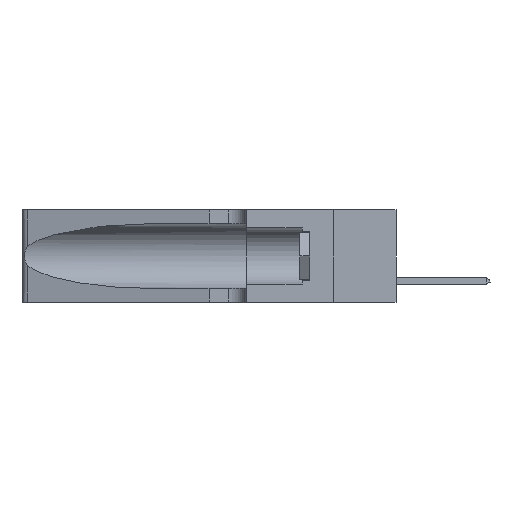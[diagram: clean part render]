
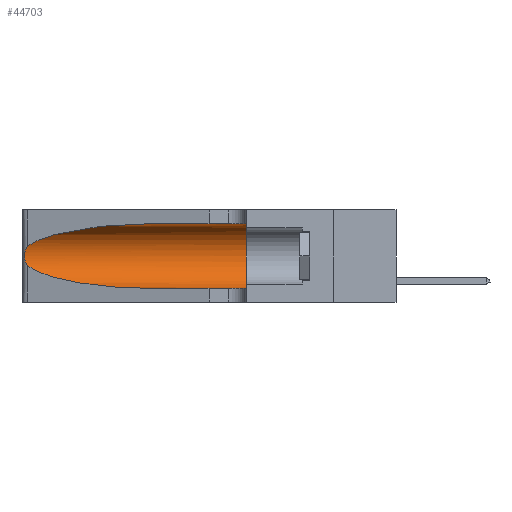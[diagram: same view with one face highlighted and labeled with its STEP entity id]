
A CAD part, left-side view. The second image highlights one B-rep face of the part: STEP entity #44703.
In plain terms, the highlighted cylindrical face has radius 3.308 mm (diameter 6.617 mm), a partial arc.
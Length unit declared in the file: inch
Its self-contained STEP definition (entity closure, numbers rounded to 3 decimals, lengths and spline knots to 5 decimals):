
#1345 = CARTESIAN_POINT ( 'NONE',  ( 0.1305, 1.61858, 0.31525 ) ) ;
#1456 = VECTOR ( 'NONE', #12982, 39.37008 ) ;
#1526 = LINE ( 'NONE', #47453, #8166 ) ;
#2474 = CARTESIAN_POINT ( 'NONE',  ( 0.18966, 0.96281, 0.05475 ) ) ;
#3058 = EDGE_CURVE ( 'NONE', #39833, #16531, #39866, .T. ) ;
#3424 = CARTESIAN_POINT ( 'NONE',  ( 0.26075, 1.23896, 0.19203 ) ) ;
#3947 = CARTESIAN_POINT ( 'NONE',  ( 0.1305, 0.35, 0.31525 ) ) ;
#3964 =( BOUNDED_CURVE ( )  B_SPLINE_CURVE ( 3, ( #33875, #34039, #11631, #26114 ),
 .UNSPECIFIED., .F., .F. ) 
 B_SPLINE_CURVE_WITH_KNOTS ( ( 4, 4 ),
 ( 1.5708, 2.84003 ),
 .UNSPECIFIED. ) 
 CURVE ( )  GEOMETRIC_REPRESENTATION_ITEM ( )  RATIONAL_B_SPLINE_CURVE ( ( 1., 0.87, 0.87, 1. ) ) 
 REPRESENTATION_ITEM ( '' )  );
#5679 = VERTEX_POINT ( 'NONE', #9797 ) ;
#6793 = FACE_OUTER_BOUND ( 'NONE', #22926, .T. ) ;
#7831 = CARTESIAN_POINT ( 'NONE',  ( 0.25787, 1.23484, 0.2124 ) ) ;
#8166 = VECTOR ( 'NONE', #40306, 39.37008 ) ;
#9797 = CARTESIAN_POINT ( 'NONE',  ( 0.1305, 0.72297, 0.31525 ) ) ;
#9865 = VERTEX_POINT ( 'NONE', #22354 ) ;
#11631 = CARTESIAN_POINT ( 'NONE',  ( 0.2373, 1.15595, 0.28018 ) ) ;
#11641 = CARTESIAN_POINT ( 'NONE',  ( 0.25854, 1.2359, 0.20912 ) ) ;
#11801 = CARTESIAN_POINT ( 'NONE',  ( 0.25555, 1.22993, 0.14849 ) ) ;
#12735 = CARTESIAN_POINT ( 'NONE',  ( 0.25487, 1.22718, 0.14631 ) ) ;
#12982 = DIRECTION ( 'NONE',  ( 0., -1., 0. ) ) ;
#15168 = DIRECTION ( 'NONE',  ( 0., 0., -1. ) ) ;
#15438 = CARTESIAN_POINT ( 'NONE',  ( 0.25789, 1.23486, 0.15765 ) ) ;
#15832 = VERTEX_POINT ( 'NONE', #45997 ) ;
#15910 = CARTESIAN_POINT ( 'NONE',  ( 0.26017, 1.23833, 0.17102 ) ) ;
#16397 = B_SPLINE_CURVE_WITH_KNOTS ( 'NONE', 3,
 ( #17649, #21635, #41900, #7831, #11641, #18788, #3424, #42201, #15910, #34995, #15438, #26889, #11801, #12735 ),
 .UNSPECIFIED., .F., .F.,
 ( 4, 2, 2, 2, 2, 2, 4 ),
 ( 0., 0.00027, 0.00053, 0.00107, 0.0016, 0.00187, 0.00214 ),
 .UNSPECIFIED. ) ;
#16531 = VERTEX_POINT ( 'NONE', #26432 ) ;
#16552 = CARTESIAN_POINT ( 'NONE',  ( 0.1305, 0.35, 0.185 ) ) ;
#16793 = CYLINDRICAL_SURFACE ( 'NONE', #22483, 0.13025 ) ;
#17649 = CARTESIAN_POINT ( 'NONE',  ( 0.25487, 1.22718, 0.22369 ) ) ;
#17921 =( BOUNDED_CURVE ( )  B_SPLINE_CURVE ( 3, ( #32791, #21204, #2474, #32284 ),
 .UNSPECIFIED., .F., .F. ) 
 B_SPLINE_CURVE_WITH_KNOTS ( ( 4, 4 ),
 ( 3.44316, 4.71239 ),
 .UNSPECIFIED. ) 
 CURVE ( )  GEOMETRIC_REPRESENTATION_ITEM ( )  RATIONAL_B_SPLINE_CURVE ( ( 1., 0.87, 0.87, 1. ) ) 
 REPRESENTATION_ITEM ( '' )  );
#18788 = CARTESIAN_POINT ( 'NONE',  ( 0.26018, 1.23835, 0.19895 ) ) ;
#19609 = EDGE_CURVE ( 'NONE', #5679, #15832, #3964, .T. ) ;
#20183 = VERTEX_POINT ( 'NONE', #21693 ) ;
#20194 = ORIENTED_EDGE ( 'NONE', *, *, #19609, .T. ) ;
#21204 = CARTESIAN_POINT ( 'NONE',  ( 0.2373, 1.15595, 0.08982 ) ) ;
#21635 = CARTESIAN_POINT ( 'NONE',  ( 0.25555, 1.22994, 0.2215 ) ) ;
#21693 = CARTESIAN_POINT ( 'NONE',  ( 0.1305, 0.72297, 0.05475 ) ) ;
#22354 = CARTESIAN_POINT ( 'NONE',  ( 0.25487, 1.22718, 0.14631 ) ) ;
#22483 = AXIS2_PLACEMENT_3D ( 'NONE', #34413, #46267, #15168 ) ;
#22926 = EDGE_LOOP ( 'NONE', ( #20194, #25824, #36470, #25529, #37662, #26844 ) ) ;
#25529 = ORIENTED_EDGE ( 'NONE', *, *, #39795, .T. ) ;
#25824 = ORIENTED_EDGE ( 'NONE', *, *, #34893, .T. ) ;
#26114 = CARTESIAN_POINT ( 'NONE',  ( 0.25487, 1.22718, 0.22369 ) ) ;
#26432 = CARTESIAN_POINT ( 'NONE',  ( 0.1305, 0.35, 0.05475 ) ) ;
#26844 = ORIENTED_EDGE ( 'NONE', *, *, #29515, .F. ) ;
#26889 = CARTESIAN_POINT ( 'NONE',  ( 0.25639, 1.23186, 0.15144 ) ) ;
#27024 = AXIS2_PLACEMENT_3D ( 'NONE', #16552, #31777, #46833 ) ;
#29515 = EDGE_CURVE ( 'NONE', #5679, #39833, #31720, .T. ) ;
#31720 = LINE ( 'NONE', #1345, #1456 ) ;
#31777 = DIRECTION ( 'NONE',  ( 0., 1., 0. ) ) ;
#32284 = CARTESIAN_POINT ( 'NONE',  ( 0.1305, 0.72297, 0.05475 ) ) ;
#32791 = CARTESIAN_POINT ( 'NONE',  ( 0.25487, 1.22718, 0.14631 ) ) ;
#33875 = CARTESIAN_POINT ( 'NONE',  ( 0.1305, 0.72297, 0.31525 ) ) ;
#34039 = CARTESIAN_POINT ( 'NONE',  ( 0.18966, 0.96281, 0.31525 ) ) ;
#34413 = CARTESIAN_POINT ( 'NONE',  ( 0.1305, 1.61858, 0.185 ) ) ;
#34893 = EDGE_CURVE ( 'NONE', #15832, #9865, #16397, .T. ) ;
#34995 = CARTESIAN_POINT ( 'NONE',  ( 0.25856, 1.23593, 0.16098 ) ) ;
#36470 = ORIENTED_EDGE ( 'NONE', *, *, #48882, .T. ) ;
#37662 = ORIENTED_EDGE ( 'NONE', *, *, #3058, .F. ) ;
#39795 = EDGE_CURVE ( 'NONE', #20183, #16531, #1526, .T. ) ;
#39833 = VERTEX_POINT ( 'NONE', #3947 ) ;
#39866 = CIRCLE ( 'NONE', #27024, 0.13025 ) ;
#40306 = DIRECTION ( 'NONE',  ( 0., -1., 0. ) ) ;
#41900 = CARTESIAN_POINT ( 'NONE',  ( 0.25639, 1.23184, 0.21858 ) ) ;
#42201 = CARTESIAN_POINT ( 'NONE',  ( 0.26075, 1.23896, 0.178 ) ) ;
#44703 = ADVANCED_FACE ( 'NONE', ( #6793 ), #16793, .F. ) ;
#45997 = CARTESIAN_POINT ( 'NONE',  ( 0.25487, 1.22718, 0.22369 ) ) ;
#46267 = DIRECTION ( 'NONE',  ( 0., -1., 0. ) ) ;
#46833 = DIRECTION ( 'NONE',  ( 0., 0., 1. ) ) ;
#47453 = CARTESIAN_POINT ( 'NONE',  ( 0.1305, 1.61858, 0.05475 ) ) ;
#48882 = EDGE_CURVE ( 'NONE', #9865, #20183, #17921, .T. ) ;
